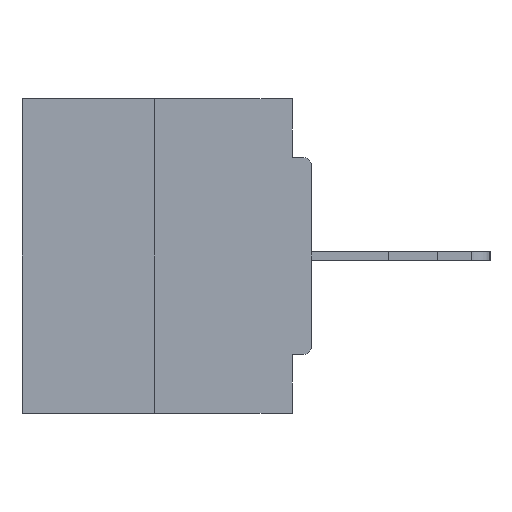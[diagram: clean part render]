
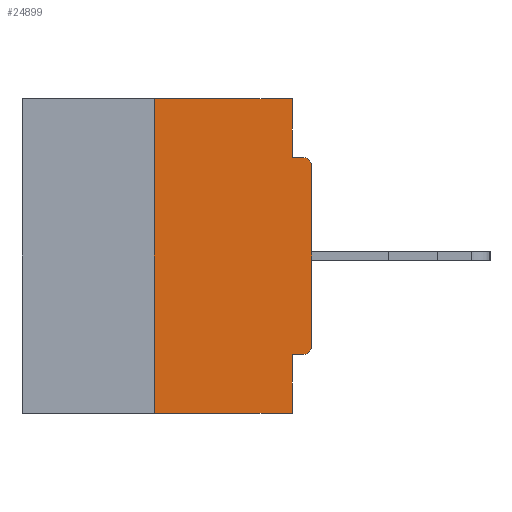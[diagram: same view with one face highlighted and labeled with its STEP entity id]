
A CAD part, left-side view. The second image highlights one B-rep face of the part: STEP entity #24899.
In plain terms, the highlighted planar face has unit normal (-1, 0, 0).
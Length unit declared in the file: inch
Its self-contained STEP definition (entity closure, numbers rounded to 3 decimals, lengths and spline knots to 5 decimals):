
#92 = AXIS2_PLACEMENT_3D ( 'NONE', #27357, #15328, #3277 ) ;
#491 = ORIENTED_EDGE ( 'NONE', *, *, #13300, .T. ) ;
#595 = CARTESIAN_POINT ( 'NONE',  ( 0., 0.031, -0.5 ) ) ;
#1594 = CIRCLE ( 'NONE', #92, 0.015 ) ;
#1799 = CARTESIAN_POINT ( 'NONE',  ( 0., 0.25, -0.5 ) ) ;
#2575 = DIRECTION ( 'NONE',  ( -1., 0., 0. ) ) ;
#2607 = VERTEX_POINT ( 'NONE', #26504 ) ;
#2852 = CARTESIAN_POINT ( 'NONE',  ( 0., 0., -0.4065 ) ) ;
#3277 = DIRECTION ( 'NONE',  ( 0., 0., -1. ) ) ;
#3453 = LINE ( 'NONE', #3607, #8700 ) ;
#3528 = EDGE_CURVE ( 'NONE', #29609, #21319, #1594, .T. ) ;
#3576 = CARTESIAN_POINT ( 'NONE',  ( 0., 0.031, 0. ) ) ;
#3607 = CARTESIAN_POINT ( 'NONE',  ( 0., 0., 0. ) ) ;
#3836 = CIRCLE ( 'NONE', #29860, 0.015 ) ;
#3961 = LINE ( 'NONE', #25705, #12769 ) ;
#4566 = LINE ( 'NONE', #6763, #19156 ) ;
#4932 = VERTEX_POINT ( 'NONE', #25791 ) ;
#5167 = CARTESIAN_POINT ( 'NONE',  ( 0., 0.46, -0.5 ) ) ;
#5293 = CARTESIAN_POINT ( 'NONE',  ( 0., 0.46, 0. ) ) ;
#5416 = ORIENTED_EDGE ( 'NONE', *, *, #10186, .T. ) ;
#6372 = VECTOR ( 'NONE', #20470, 39.37008 ) ;
#6763 = CARTESIAN_POINT ( 'NONE',  ( 0., 0., -0.0935 ) ) ;
#7278 = CARTESIAN_POINT ( 'NONE',  ( 0., 0.015, -0.3915 ) ) ;
#7381 = ORIENTED_EDGE ( 'NONE', *, *, #21575, .F. ) ;
#7761 = CARTESIAN_POINT ( 'NONE',  ( 0., 0.031, 0. ) ) ;
#8632 = LINE ( 'NONE', #25660, #17703 ) ;
#8700 = VECTOR ( 'NONE', #13139, 39.37008 ) ;
#9753 = CARTESIAN_POINT ( 'NONE',  ( 0., 0., -0.3915 ) ) ;
#9817 = EDGE_CURVE ( 'NONE', #2607, #4932, #26933, .T. ) ;
#10186 = EDGE_CURVE ( 'NONE', #14779, #21129, #26742, .T. ) ;
#10973 = DIRECTION ( 'NONE',  ( 0., 0., 1. ) ) ;
#11088 = LINE ( 'NONE', #3576, #6372 ) ;
#11149 = DIRECTION ( 'NONE',  ( 0., -1., 0. ) ) ;
#11810 = VERTEX_POINT ( 'NONE', #14561 ) ;
#12063 = ORIENTED_EDGE ( 'NONE', *, *, #24948, .F. ) ;
#12769 = VECTOR ( 'NONE', #27883, 39.37008 ) ;
#12887 = ORIENTED_EDGE ( 'NONE', *, *, #9817, .F. ) ;
#13139 = DIRECTION ( 'NONE',  ( 0., 0., 1. ) ) ;
#13300 = EDGE_CURVE ( 'NONE', #29997, #29609, #3453, .T. ) ;
#14321 = CARTESIAN_POINT ( 'NONE',  ( 0., 0., -0.1085 ) ) ;
#14561 = CARTESIAN_POINT ( 'NONE',  ( 0., 0.031, -0.0935 ) ) ;
#14779 = VERTEX_POINT ( 'NONE', #1799 ) ;
#14832 = DIRECTION ( 'NONE',  ( 0., 0., -1. ) ) ;
#15328 = DIRECTION ( 'NONE',  ( -1., 0., 0. ) ) ;
#15457 = VECTOR ( 'NONE', #22056, 39.37008 ) ;
#16526 = EDGE_CURVE ( 'NONE', #4932, #21129, #3961, .T. ) ;
#16946 = CARTESIAN_POINT ( 'NONE',  ( 0., 0.015, -0.0935 ) ) ;
#17702 = VECTOR ( 'NONE', #25756, 39.37008 ) ;
#17703 = VECTOR ( 'NONE', #10973, 39.37008 ) ;
#17942 = LINE ( 'NONE', #21066, #17702 ) ;
#18595 = VERTEX_POINT ( 'NONE', #26199 ) ;
#19151 = ORIENTED_EDGE ( 'NONE', *, *, #28400, .T. ) ;
#19156 = VECTOR ( 'NONE', #11149, 39.37008 ) ;
#20325 = EDGE_LOOP ( 'NONE', ( #12063, #21062, #5416, #27893, #12887, #19151, #491, #30046, #7381, #26979 ) ) ;
#20470 = DIRECTION ( 'NONE',  ( 0., 0., -1. ) ) ;
#21062 = ORIENTED_EDGE ( 'NONE', *, *, #22840, .F. ) ;
#21066 = CARTESIAN_POINT ( 'NONE',  ( 0., 0.46, 0. ) ) ;
#21129 = VERTEX_POINT ( 'NONE', #595 ) ;
#21319 = VERTEX_POINT ( 'NONE', #16946 ) ;
#21575 = EDGE_CURVE ( 'NONE', #11810, #21319, #4566, .T. ) ;
#22056 = DIRECTION ( 'NONE',  ( 0., -1., 0. ) ) ;
#22643 = FACE_OUTER_BOUND ( 'NONE', #20325, .T. ) ;
#22840 = EDGE_CURVE ( 'NONE', #14779, #18595, #8632, .T. ) ;
#24601 = DIRECTION ( 'NONE',  ( 0., 1., 0. ) ) ;
#24689 = DIRECTION ( 'NONE',  ( 1., 0., 0. ) ) ;
#24899 = ADVANCED_FACE ( 'NONE', ( #22643 ), #24987, .F. ) ;
#24948 = EDGE_CURVE ( 'NONE', #18595, #30740, #17942, .T. ) ;
#24987 = PLANE ( 'NONE',  #28187 ) ;
#25660 = CARTESIAN_POINT ( 'NONE',  ( 0., 0.25, 0. ) ) ;
#25705 = CARTESIAN_POINT ( 'NONE',  ( 0., 0.031, -0.5 ) ) ;
#25756 = DIRECTION ( 'NONE',  ( 0., -1., 0. ) ) ;
#25791 = CARTESIAN_POINT ( 'NONE',  ( 0., 0.031, -0.4065 ) ) ;
#26199 = CARTESIAN_POINT ( 'NONE',  ( 0., 0.25, 0. ) ) ;
#26504 = CARTESIAN_POINT ( 'NONE',  ( 0., 0.015, -0.4065 ) ) ;
#26505 = DIRECTION ( 'NONE',  ( 0., 0., -1. ) ) ;
#26742 = LINE ( 'NONE', #5167, #15457 ) ;
#26933 = LINE ( 'NONE', #2852, #27919 ) ;
#26979 = ORIENTED_EDGE ( 'NONE', *, *, #27734, .F. ) ;
#27357 = CARTESIAN_POINT ( 'NONE',  ( 0., 0.015, -0.1085 ) ) ;
#27734 = EDGE_CURVE ( 'NONE', #30740, #11810, #11088, .T. ) ;
#27883 = DIRECTION ( 'NONE',  ( 0., 0., -1. ) ) ;
#27893 = ORIENTED_EDGE ( 'NONE', *, *, #16526, .F. ) ;
#27919 = VECTOR ( 'NONE', #24601, 39.37008 ) ;
#28187 = AXIS2_PLACEMENT_3D ( 'NONE', #5293, #24689, #14832 ) ;
#28400 = EDGE_CURVE ( 'NONE', #2607, #29997, #3836, .T. ) ;
#29609 = VERTEX_POINT ( 'NONE', #14321 ) ;
#29860 = AXIS2_PLACEMENT_3D ( 'NONE', #7278, #2575, #26505 ) ;
#29997 = VERTEX_POINT ( 'NONE', #9753 ) ;
#30046 = ORIENTED_EDGE ( 'NONE', *, *, #3528, .T. ) ;
#30740 = VERTEX_POINT ( 'NONE', #7761 ) ;
